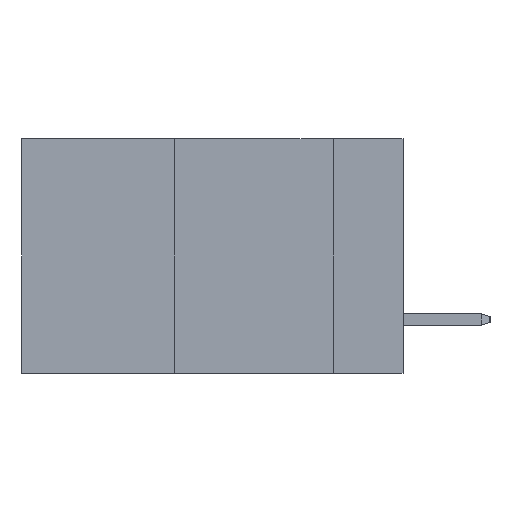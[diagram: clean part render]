
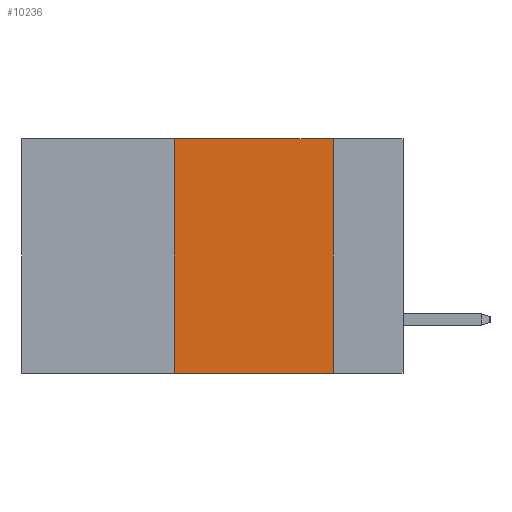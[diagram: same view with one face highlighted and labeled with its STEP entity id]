
A CAD part, left-side view. The second image highlights one B-rep face of the part: STEP entity #10236.
In plain terms, the highlighted planar face has unit normal (-1, 0, 0).
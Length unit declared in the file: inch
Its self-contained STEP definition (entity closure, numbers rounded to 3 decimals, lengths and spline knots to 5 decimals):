
#535 = CARTESIAN_POINT ( 'NONE',  ( 0., 0.6, 0. ) ) ;
#911 = VECTOR ( 'NONE', #6441, 39.37008 ) ;
#1125 = EDGE_CURVE ( 'NONE', #3604, #12926, #12837, .T. ) ;
#1596 = DIRECTION ( 'NONE',  ( 0., 0., -1. ) ) ;
#1862 = FACE_OUTER_BOUND ( 'NONE', #12004, .T. ) ;
#2032 = DIRECTION ( 'NONE',  ( 0., -1., 0. ) ) ;
#2461 = CARTESIAN_POINT ( 'NONE',  ( 0., 0.36, 0. ) ) ;
#2834 = ORIENTED_EDGE ( 'NONE', *, *, #1125, .T. ) ;
#3381 = VERTEX_POINT ( 'NONE', #8186 ) ;
#3604 = VERTEX_POINT ( 'NONE', #5697 ) ;
#3894 = VECTOR ( 'NONE', #8804, 39.37008 ) ;
#4180 = LINE ( 'NONE', #7288, #5407 ) ;
#4195 = DIRECTION ( 'NONE',  ( 0., 0., -1. ) ) ;
#4333 = LINE ( 'NONE', #2461, #911 ) ;
#4571 = ORIENTED_EDGE ( 'NONE', *, *, #8696, .F. ) ;
#5407 = VECTOR ( 'NONE', #2032, 39.37008 ) ;
#5436 = AXIS2_PLACEMENT_3D ( 'NONE', #535, #8740, #1596 ) ;
#5697 = CARTESIAN_POINT ( 'NONE',  ( 0., 0.36, -0.37 ) ) ;
#5978 = PLANE ( 'NONE',  #5436 ) ;
#6441 = DIRECTION ( 'NONE',  ( 0., 0., 1. ) ) ;
#6617 = VERTEX_POINT ( 'NONE', #13281 ) ;
#6718 = CARTESIAN_POINT ( 'NONE',  ( 0., 0.6, -0.37 ) ) ;
#7288 = CARTESIAN_POINT ( 'NONE',  ( 0., 0.6, 0. ) ) ;
#8186 = CARTESIAN_POINT ( 'NONE',  ( 0., 0.11, 0. ) ) ;
#8246 = VECTOR ( 'NONE', #4195, 39.37008 ) ;
#8696 = EDGE_CURVE ( 'NONE', #6617, #3381, #4180, .T. ) ;
#8740 = DIRECTION ( 'NONE',  ( 1., 0., 0. ) ) ;
#8804 = DIRECTION ( 'NONE',  ( 0., -1., 0. ) ) ;
#9018 = CARTESIAN_POINT ( 'NONE',  ( 0., 0.11, -0.37 ) ) ;
#9198 = EDGE_CURVE ( 'NONE', #3604, #6617, #4333, .T. ) ;
#10137 = CARTESIAN_POINT ( 'NONE',  ( 0., 0.11, 0. ) ) ;
#10206 = LINE ( 'NONE', #10137, #8246 ) ;
#10236 = ADVANCED_FACE ( 'NONE', ( #1862 ), #5978, .F. ) ;
#10340 = EDGE_CURVE ( 'NONE', #3381, #12926, #10206, .T. ) ;
#11846 = ORIENTED_EDGE ( 'NONE', *, *, #9198, .F. ) ;
#12004 = EDGE_LOOP ( 'NONE', ( #12336, #4571, #11846, #2834 ) ) ;
#12336 = ORIENTED_EDGE ( 'NONE', *, *, #10340, .F. ) ;
#12837 = LINE ( 'NONE', #6718, #3894 ) ;
#12926 = VERTEX_POINT ( 'NONE', #9018 ) ;
#13281 = CARTESIAN_POINT ( 'NONE',  ( 0., 0.36, 0. ) ) ;
